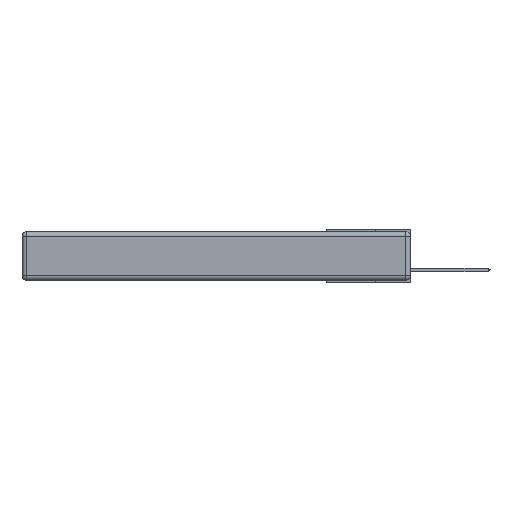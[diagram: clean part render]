
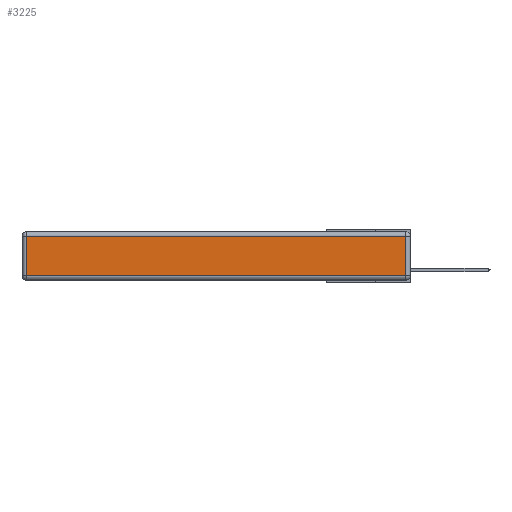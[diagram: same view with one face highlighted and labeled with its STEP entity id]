
A CAD part, left-side view. The second image highlights one B-rep face of the part: STEP entity #3225.
In plain terms, the highlighted planar face has unit normal (-1, 0, 0).
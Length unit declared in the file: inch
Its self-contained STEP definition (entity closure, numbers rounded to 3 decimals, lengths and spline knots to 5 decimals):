
#81 = LINE ( 'NONE', #13101, #438 ) ;
#85 = EDGE_LOOP ( 'NONE', ( #1063, #15152, #7774, #11335 ) ) ;
#438 = VECTOR ( 'NONE', #9692, 39.37008 ) ;
#1063 = ORIENTED_EDGE ( 'NONE', *, *, #12456, .T. ) ;
#1356 = CARTESIAN_POINT ( 'NONE',  ( 0., 0.03, -0.313 ) ) ;
#1635 = FACE_OUTER_BOUND ( 'NONE', #85, .T. ) ;
#1966 = LINE ( 'NONE', #2994, #10779 ) ;
#2245 = LINE ( 'NONE', #11068, #7886 ) ;
#2281 = VERTEX_POINT ( 'NONE', #1356 ) ;
#2897 = DIRECTION ( 'NONE',  ( -1., 0., 0. ) ) ;
#2994 = CARTESIAN_POINT ( 'NONE',  ( 0., 2.75, -0.03 ) ) ;
#3225 = ADVANCED_FACE ( 'NONE', ( #1635 ), #5548, .T. ) ;
#4020 = CARTESIAN_POINT ( 'NONE',  ( 0., 2.72, -0.313 ) ) ;
#4344 = CARTESIAN_POINT ( 'NONE',  ( 0., 2.72, -0.343 ) ) ;
#5234 = DIRECTION ( 'NONE',  ( 0., -1., 0. ) ) ;
#5296 = EDGE_CURVE ( 'NONE', #10633, #13654, #1966, .T. ) ;
#5548 = PLANE ( 'NONE',  #5566 ) ;
#5566 = AXIS2_PLACEMENT_3D ( 'NONE', #13770, #2897, #6764 ) ;
#5751 = LINE ( 'NONE', #4344, #10020 ) ;
#6764 = DIRECTION ( 'NONE',  ( 0., 0., 1. ) ) ;
#7774 = ORIENTED_EDGE ( 'NONE', *, *, #5296, .T. ) ;
#7886 = VECTOR ( 'NONE', #5234, 39.37008 ) ;
#8979 = DIRECTION ( 'NONE',  ( 0., 1., 0. ) ) ;
#9407 = VERTEX_POINT ( 'NONE', #4020 ) ;
#9692 = DIRECTION ( 'NONE',  ( 0., 0., 1. ) ) ;
#9951 = EDGE_CURVE ( 'NONE', #13654, #9407, #5751, .T. ) ;
#10020 = VECTOR ( 'NONE', #11655, 39.37008 ) ;
#10633 = VERTEX_POINT ( 'NONE', #11224 ) ;
#10779 = VECTOR ( 'NONE', #8979, 39.37008 ) ;
#11068 = CARTESIAN_POINT ( 'NONE',  ( 0., 0., -0.313 ) ) ;
#11224 = CARTESIAN_POINT ( 'NONE',  ( 0., 0.03, -0.03 ) ) ;
#11335 = ORIENTED_EDGE ( 'NONE', *, *, #9951, .T. ) ;
#11642 = CARTESIAN_POINT ( 'NONE',  ( 0., 2.72, -0.03 ) ) ;
#11655 = DIRECTION ( 'NONE',  ( 0., 0., -1. ) ) ;
#12456 = EDGE_CURVE ( 'NONE', #9407, #2281, #2245, .T. ) ;
#13101 = CARTESIAN_POINT ( 'NONE',  ( 0., 0.03, -0.343 ) ) ;
#13654 = VERTEX_POINT ( 'NONE', #11642 ) ;
#13770 = CARTESIAN_POINT ( 'NONE',  ( 0., 0., -0.343 ) ) ;
#15152 = ORIENTED_EDGE ( 'NONE', *, *, #15243, .T. ) ;
#15243 = EDGE_CURVE ( 'NONE', #2281, #10633, #81, .T. ) ;
